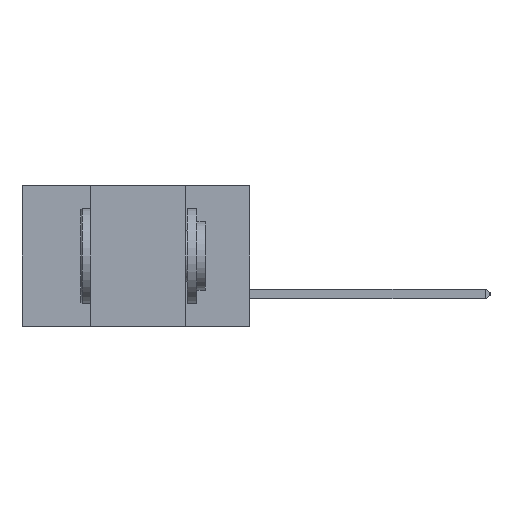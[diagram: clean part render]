
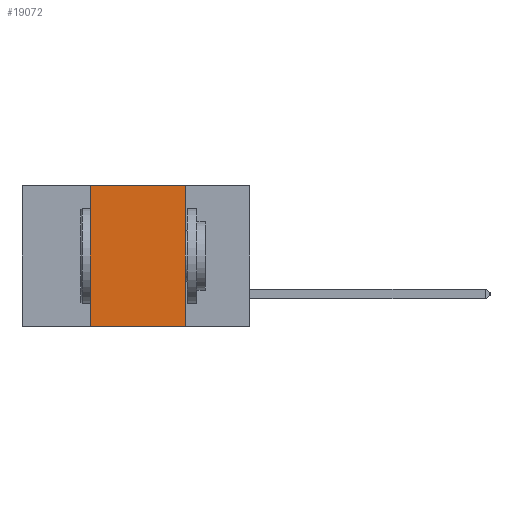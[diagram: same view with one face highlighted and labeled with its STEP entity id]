
A CAD part, left-side view. The second image highlights one B-rep face of the part: STEP entity #19072.
In plain terms, the highlighted planar face has unit normal (-1, 0, 0).
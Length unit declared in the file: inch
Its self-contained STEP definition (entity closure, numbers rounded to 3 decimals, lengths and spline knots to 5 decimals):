
#2627 = CARTESIAN_POINT ( 'NONE',  ( 0., 0.42, -0.37 ) ) ;
#2904 = EDGE_CURVE ( 'NONE', #12064, #19581, #10514, .T. ) ;
#3216 = ORIENTED_EDGE ( 'NONE', *, *, #12332, .F. ) ;
#5441 = AXIS2_PLACEMENT_3D ( 'NONE', #8146, #9935, #21878 ) ;
#5838 = VECTOR ( 'NONE', #9297, 39.37008 ) ;
#6407 = PLANE ( 'NONE',  #5441 ) ;
#7028 = VECTOR ( 'NONE', #9482, 39.37008 ) ;
#8146 = CARTESIAN_POINT ( 'NONE',  ( 0., 0.6, 0. ) ) ;
#8647 = CARTESIAN_POINT ( 'NONE',  ( 0., 0.42, 0. ) ) ;
#9297 = DIRECTION ( 'NONE',  ( 0., -1., 0. ) ) ;
#9335 = EDGE_LOOP ( 'NONE', ( #14931, #20250, #3216, #13622 ) ) ;
#9482 = DIRECTION ( 'NONE',  ( 0., -1., 0. ) ) ;
#9642 = CARTESIAN_POINT ( 'NONE',  ( 0., 0.17, 0. ) ) ;
#9666 = CARTESIAN_POINT ( 'NONE',  ( 0., 0.6, -0.37 ) ) ;
#9846 = DIRECTION ( 'NONE',  ( 0., 0., -1. ) ) ;
#9935 = DIRECTION ( 'NONE',  ( 1., 0., 0. ) ) ;
#10424 = DIRECTION ( 'NONE',  ( 0., 0., 1. ) ) ;
#10498 = LINE ( 'NONE', #8647, #19064 ) ;
#10514 = LINE ( 'NONE', #9666, #5838 ) ;
#10546 = EDGE_CURVE ( 'NONE', #12665, #18457, #11651, .T. ) ;
#11651 = LINE ( 'NONE', #19737, #7028 ) ;
#11714 = LINE ( 'NONE', #16691, #20255 ) ;
#12064 = VERTEX_POINT ( 'NONE', #2627 ) ;
#12332 = EDGE_CURVE ( 'NONE', #12064, #12665, #10498, .T. ) ;
#12665 = VERTEX_POINT ( 'NONE', #21518 ) ;
#13622 = ORIENTED_EDGE ( 'NONE', *, *, #2904, .T. ) ;
#14733 = CARTESIAN_POINT ( 'NONE',  ( 0., 0.17, -0.37 ) ) ;
#14931 = ORIENTED_EDGE ( 'NONE', *, *, #19038, .F. ) ;
#16261 = FACE_OUTER_BOUND ( 'NONE', #9335, .T. ) ;
#16691 = CARTESIAN_POINT ( 'NONE',  ( 0., 0.17, 0. ) ) ;
#18457 = VERTEX_POINT ( 'NONE', #9642 ) ;
#19038 = EDGE_CURVE ( 'NONE', #18457, #19581, #11714, .T. ) ;
#19064 = VECTOR ( 'NONE', #10424, 39.37008 ) ;
#19072 = ADVANCED_FACE ( 'NONE', ( #16261 ), #6407, .F. ) ;
#19581 = VERTEX_POINT ( 'NONE', #14733 ) ;
#19737 = CARTESIAN_POINT ( 'NONE',  ( 0., 0.6, 0. ) ) ;
#20250 = ORIENTED_EDGE ( 'NONE', *, *, #10546, .F. ) ;
#20255 = VECTOR ( 'NONE', #9846, 39.37008 ) ;
#21518 = CARTESIAN_POINT ( 'NONE',  ( 0., 0.42, 0. ) ) ;
#21878 = DIRECTION ( 'NONE',  ( 0., 0., -1. ) ) ;
